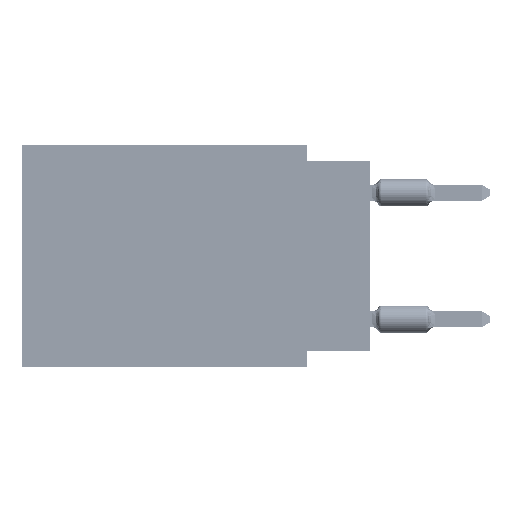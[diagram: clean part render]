
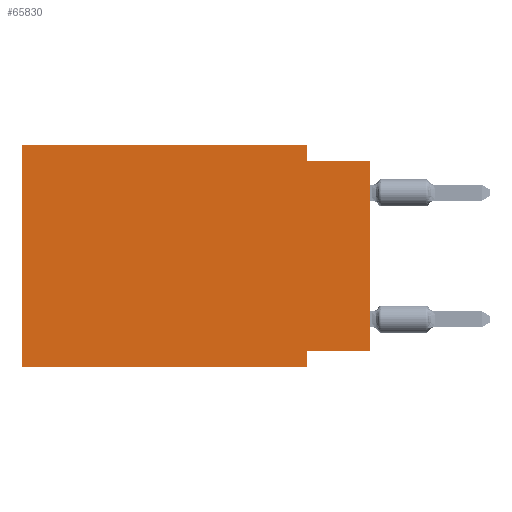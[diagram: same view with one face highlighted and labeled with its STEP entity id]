
A CAD part, left-side view. The second image highlights one B-rep face of the part: STEP entity #65830.
In plain terms, the highlighted planar face has unit normal (-1, 0, 0).
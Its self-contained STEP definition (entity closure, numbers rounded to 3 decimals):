
#1704 = EDGE_CURVE ( 'NONE', #10596, #68548, #23093, .T. ) ;
#5214 = LINE ( 'NONE', #70989, #10695 ) ;
#5389 = DIRECTION ( 'NONE',  ( 0., -1., 0. ) ) ;
#5641 = DIRECTION ( 'NONE',  ( 0., -1., 0. ) ) ;
#7075 = VERTEX_POINT ( 'NONE', #19187 ) ;
#7529 = DIRECTION ( 'NONE',  ( 0., 0., -1. ) ) ;
#8523 = CARTESIAN_POINT ( 'NONE',  ( 0., 13.97, 0. ) ) ;
#8668 = CARTESIAN_POINT ( 'NONE',  ( 0., 13.97, -8.89 ) ) ;
#10596 = VERTEX_POINT ( 'NONE', #8668 ) ;
#10695 = VECTOR ( 'NONE', #95765, 1000. ) ;
#11407 = DIRECTION ( 'NONE',  ( 0., -1., 0. ) ) ;
#11928 = CARTESIAN_POINT ( 'NONE',  ( 0., 13.97, 0. ) ) ;
#13119 = CARTESIAN_POINT ( 'NONE',  ( 0., 0., -8.255 ) ) ;
#19187 = CARTESIAN_POINT ( 'NONE',  ( 0., 0., -0.635 ) ) ;
#21275 = CARTESIAN_POINT ( 'NONE',  ( 0., 13.97, 0. ) ) ;
#21810 = CARTESIAN_POINT ( 'NONE',  ( 0., 13.97, 0. ) ) ;
#23093 = LINE ( 'NONE', #8523, #88468 ) ;
#23359 = CARTESIAN_POINT ( 'NONE',  ( 0., 2.54, -8.255 ) ) ;
#26760 = CARTESIAN_POINT ( 'NONE',  ( 0., 2.54, 0. ) ) ;
#27036 = CARTESIAN_POINT ( 'NONE',  ( 0., 13.97, -8.89 ) ) ;
#30432 = LINE ( 'NONE', #21810, #48097 ) ;
#30574 = LINE ( 'NONE', #31109, #56423 ) ;
#31109 = CARTESIAN_POINT ( 'NONE',  ( 0., 0., 0. ) ) ;
#32289 = VERTEX_POINT ( 'NONE', #84646 ) ;
#36542 = EDGE_CURVE ( 'NONE', #50885, #93634, #55534, .T. ) ;
#41178 = EDGE_CURVE ( 'NONE', #60598, #50885, #5214, .T. ) ;
#41844 = CARTESIAN_POINT ( 'NONE',  ( 0., 2.54, -8.89 ) ) ;
#43211 = ORIENTED_EDGE ( 'NONE', *, *, #41178, .F. ) ;
#45328 = CARTESIAN_POINT ( 'NONE',  ( 0., 2.54, 0. ) ) ;
#48097 = VECTOR ( 'NONE', #5641, 1000. ) ;
#50885 = VERTEX_POINT ( 'NONE', #23359 ) ;
#55464 = DIRECTION ( 'NONE',  ( 0., 0., 1. ) ) ;
#55534 = LINE ( 'NONE', #81371, #96024 ) ;
#56423 = VECTOR ( 'NONE', #88237, 1000. ) ;
#57346 = DIRECTION ( 'NONE',  ( 0., 0., -1. ) ) ;
#60598 = VERTEX_POINT ( 'NONE', #13119 ) ;
#60727 = ORIENTED_EDGE ( 'NONE', *, *, #1704, .F. ) ;
#62182 = EDGE_LOOP ( 'NONE', ( #62481, #93960, #69212, #77316, #60727, #103411, #66202, #43211 ) ) ;
#62250 = PLANE ( 'NONE',  #101320 ) ;
#62481 = ORIENTED_EDGE ( 'NONE', *, *, #75849, .T. ) ;
#65830 = ADVANCED_FACE ( 'NONE', ( #103208 ), #62250, .F. ) ;
#66202 = ORIENTED_EDGE ( 'NONE', *, *, #36542, .F. ) ;
#68259 = DIRECTION ( 'NONE',  ( 0., 0., -1. ) ) ;
#68548 = VERTEX_POINT ( 'NONE', #11928 ) ;
#69212 = ORIENTED_EDGE ( 'NONE', *, *, #94913, .F. ) ;
#70989 = CARTESIAN_POINT ( 'NONE',  ( 0., 0., -8.255 ) ) ;
#75849 = EDGE_CURVE ( 'NONE', #60598, #7075, #30574, .T. ) ;
#76348 = LINE ( 'NONE', #26760, #89212 ) ;
#77166 = LINE ( 'NONE', #27036, #86475 ) ;
#77316 = ORIENTED_EDGE ( 'NONE', *, *, #77812, .F. ) ;
#77812 = EDGE_CURVE ( 'NONE', #68548, #85793, #30432, .T. ) ;
#77951 = EDGE_CURVE ( 'NONE', #32289, #7075, #79246, .T. ) ;
#78709 = CARTESIAN_POINT ( 'NONE',  ( 0., 0., -0.635 ) ) ;
#79246 = LINE ( 'NONE', #78709, #87667 ) ;
#81371 = CARTESIAN_POINT ( 'NONE',  ( 0., 2.54, -8.89 ) ) ;
#84646 = CARTESIAN_POINT ( 'NONE',  ( 0., 2.54, -0.635 ) ) ;
#85793 = VERTEX_POINT ( 'NONE', #45328 ) ;
#86475 = VECTOR ( 'NONE', #11407, 1000. ) ;
#86987 = EDGE_CURVE ( 'NONE', #10596, #93634, #77166, .T. ) ;
#87667 = VECTOR ( 'NONE', #5389, 1000. ) ;
#88237 = DIRECTION ( 'NONE',  ( 0., 0., 1. ) ) ;
#88468 = VECTOR ( 'NONE', #55464, 1000. ) ;
#89212 = VECTOR ( 'NONE', #68259, 1000. ) ;
#93634 = VERTEX_POINT ( 'NONE', #41844 ) ;
#93960 = ORIENTED_EDGE ( 'NONE', *, *, #77951, .F. ) ;
#94913 = EDGE_CURVE ( 'NONE', #85793, #32289, #76348, .T. ) ;
#95765 = DIRECTION ( 'NONE',  ( 0., 1., 0. ) ) ;
#96024 = VECTOR ( 'NONE', #7529, 1000. ) ;
#101320 = AXIS2_PLACEMENT_3D ( 'NONE', #21275, #103748, #57346 ) ;
#103208 = FACE_OUTER_BOUND ( 'NONE', #62182, .T. ) ;
#103411 = ORIENTED_EDGE ( 'NONE', *, *, #86987, .T. ) ;
#103748 = DIRECTION ( 'NONE',  ( 1., 0., 0. ) ) ;
